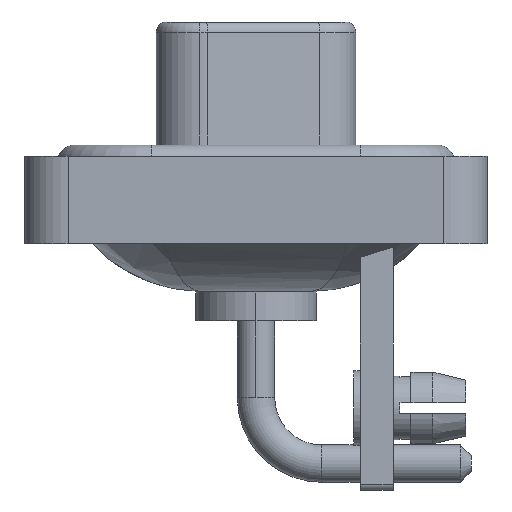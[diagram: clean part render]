
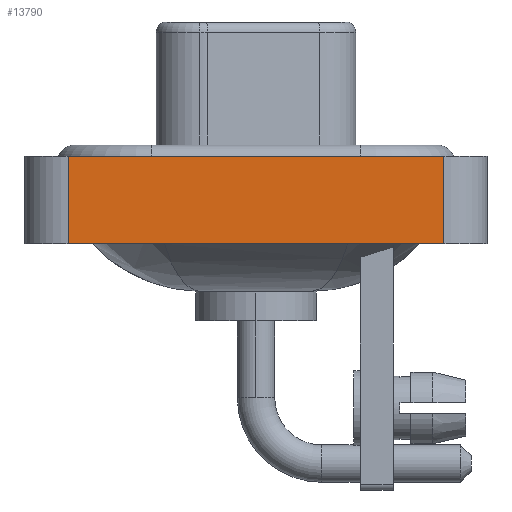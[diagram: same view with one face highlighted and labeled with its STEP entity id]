
A CAD part, left-side view. The second image highlights one B-rep face of the part: STEP entity #13790.
In plain terms, the highlighted planar face has unit normal (-1, 0, 0).
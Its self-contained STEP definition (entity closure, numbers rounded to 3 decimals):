
#401 = CARTESIAN_POINT ( 'NONE',  ( -7.25, -8.55, -3.6 ) ) ;
#2545 = LINE ( 'NONE', #6142, #6773 ) ;
#2740 = EDGE_CURVE ( 'NONE', #12586, #12028, #4696, .T. ) ;
#2869 = VECTOR ( 'NONE', #9038, 1000. ) ;
#3216 = PLANE ( 'NONE',  #4746 ) ;
#3228 = CARTESIAN_POINT ( 'NONE',  ( -7.25, 8.55, -3.6 ) ) ;
#3636 = CARTESIAN_POINT ( 'NONE',  ( -7.25, -8.55, -3.6 ) ) ;
#4585 = ORIENTED_EDGE ( 'NONE', *, *, #4971, .F. ) ;
#4696 = LINE ( 'NONE', #15647, #17428 ) ;
#4746 = AXIS2_PLACEMENT_3D ( 'NONE', #401, #5776, #8354 ) ;
#4971 = EDGE_CURVE ( 'NONE', #14845, #12028, #2545, .T. ) ;
#5049 = LINE ( 'NONE', #3636, #2869 ) ;
#5226 = CARTESIAN_POINT ( 'NONE',  ( -7.25, -8.55, 0.4 ) ) ;
#5378 = EDGE_LOOP ( 'NONE', ( #13539, #4585, #7345, #5435 ) ) ;
#5435 = ORIENTED_EDGE ( 'NONE', *, *, #5873, .T. ) ;
#5776 = DIRECTION ( 'NONE',  ( -1., 0., 0. ) ) ;
#5873 = EDGE_CURVE ( 'NONE', #10817, #12586, #5049, .T. ) ;
#6071 = CARTESIAN_POINT ( 'NONE',  ( -7.25, 8.55, 0.4 ) ) ;
#6142 = CARTESIAN_POINT ( 'NONE',  ( -7.25, -8.55, 0.4 ) ) ;
#6773 = VECTOR ( 'NONE', #16933, 1000. ) ;
#6997 = VECTOR ( 'NONE', #12566, 1000. ) ;
#7113 = FACE_OUTER_BOUND ( 'NONE', #5378, .T. ) ;
#7345 = ORIENTED_EDGE ( 'NONE', *, *, #12864, .F. ) ;
#7515 = CARTESIAN_POINT ( 'NONE',  ( -7.25, 8.55, -3.6 ) ) ;
#8354 = DIRECTION ( 'NONE',  ( 0., 0., 1. ) ) ;
#9038 = DIRECTION ( 'NONE',  ( 0., -1., 0. ) ) ;
#10817 = VERTEX_POINT ( 'NONE', #3228 ) ;
#11326 = LINE ( 'NONE', #7515, #6997 ) ;
#12028 = VERTEX_POINT ( 'NONE', #5226 ) ;
#12566 = DIRECTION ( 'NONE',  ( 0., 0., 1. ) ) ;
#12586 = VERTEX_POINT ( 'NONE', #13198 ) ;
#12839 = DIRECTION ( 'NONE',  ( 0., 0., 1. ) ) ;
#12864 = EDGE_CURVE ( 'NONE', #10817, #14845, #11326, .T. ) ;
#13198 = CARTESIAN_POINT ( 'NONE',  ( -7.25, -8.55, -3.6 ) ) ;
#13539 = ORIENTED_EDGE ( 'NONE', *, *, #2740, .T. ) ;
#13790 = ADVANCED_FACE ( 'NONE', ( #7113 ), #3216, .T. ) ;
#14845 = VERTEX_POINT ( 'NONE', #6071 ) ;
#15647 = CARTESIAN_POINT ( 'NONE',  ( -7.25, -8.55, -3.6 ) ) ;
#16933 = DIRECTION ( 'NONE',  ( 0., -1., 0. ) ) ;
#17428 = VECTOR ( 'NONE', #12839, 1000. ) ;
